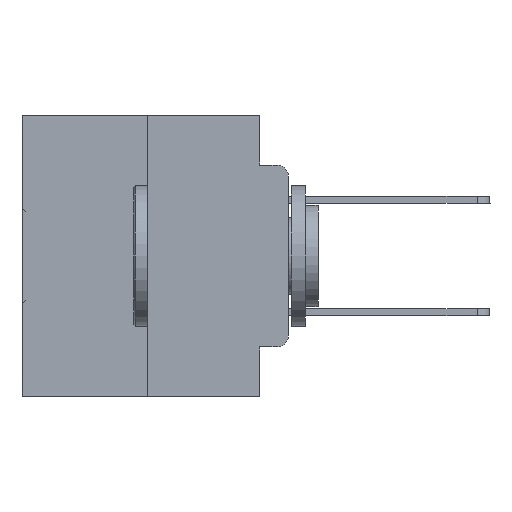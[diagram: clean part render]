
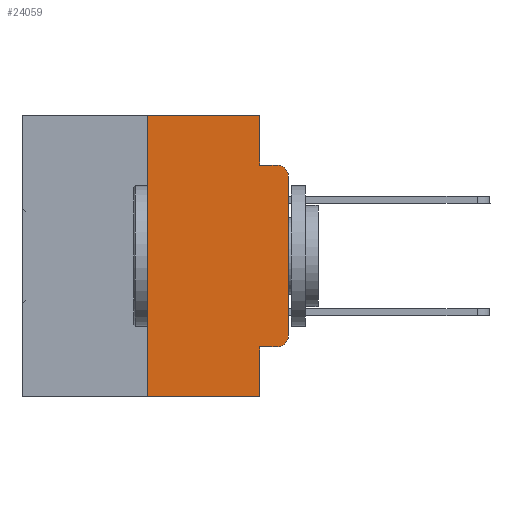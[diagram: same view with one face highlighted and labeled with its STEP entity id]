
A CAD part, left-side view. The second image highlights one B-rep face of the part: STEP entity #24059.
In plain terms, the highlighted planar face has unit normal (-1, 0, 0).
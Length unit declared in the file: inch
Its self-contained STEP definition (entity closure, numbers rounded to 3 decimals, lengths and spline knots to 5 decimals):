
#726 = EDGE_LOOP ( 'NONE', ( #24834, #34474, #28159, #8628, #19792, #15098, #16717, #9718, #22129, #34098 ) ) ;
#795 = EDGE_CURVE ( 'NONE', #1581, #10799, #4745, .T. ) ;
#1581 = VERTEX_POINT ( 'NONE', #32515 ) ;
#2024 = CARTESIAN_POINT ( 'NONE',  ( 0., 0.473, 0. ) ) ;
#2047 = DIRECTION ( 'NONE',  ( -1., 0., 0. ) ) ;
#2384 = DIRECTION ( 'NONE',  ( -1., 0., 0. ) ) ;
#2944 = DIRECTION ( 'NONE',  ( 0., -1., 0. ) ) ;
#4261 = EDGE_CURVE ( 'NONE', #22751, #6468, #29670, .T. ) ;
#4745 = LINE ( 'NONE', #30474, #30643 ) ;
#4764 = CARTESIAN_POINT ( 'NONE',  ( 0., 0.051, -0.4115 ) ) ;
#4934 = FACE_OUTER_BOUND ( 'NONE', #726, .T. ) ;
#5208 = CIRCLE ( 'NONE', #13096, 0.02 ) ;
#5862 = EDGE_CURVE ( 'NONE', #1581, #19185, #18358, .T. ) ;
#6235 = VERTEX_POINT ( 'NONE', #17191 ) ;
#6460 = CIRCLE ( 'NONE', #14103, 0.02 ) ;
#6468 = VERTEX_POINT ( 'NONE', #27040 ) ;
#6824 = EDGE_CURVE ( 'NONE', #12657, #6235, #22444, .T. ) ;
#8425 = LINE ( 'NONE', #23214, #25607 ) ;
#8628 = ORIENTED_EDGE ( 'NONE', *, *, #6824, .F. ) ;
#9556 = DIRECTION ( 'NONE',  ( 0., -1., 0. ) ) ;
#9718 = ORIENTED_EDGE ( 'NONE', *, *, #28615, .F. ) ;
#9934 = VECTOR ( 'NONE', #9556, 39.37008 ) ;
#10799 = VERTEX_POINT ( 'NONE', #25189 ) ;
#10883 = CARTESIAN_POINT ( 'NONE',  ( 0., 0.051, -0.5 ) ) ;
#11021 = CARTESIAN_POINT ( 'NONE',  ( 0., 0.473, -0.5 ) ) ;
#11937 = VECTOR ( 'NONE', #12017, 39.37008 ) ;
#12017 = DIRECTION ( 'NONE',  ( 0., 0., -1. ) ) ;
#12071 = DIRECTION ( 'NONE',  ( 0., -1., 0. ) ) ;
#12657 = VERTEX_POINT ( 'NONE', #19459 ) ;
#12986 = LINE ( 'NONE', #22172, #19304 ) ;
#13096 = AXIS2_PLACEMENT_3D ( 'NONE', #21367, #2384, #29260 ) ;
#14103 = AXIS2_PLACEMENT_3D ( 'NONE', #23578, #2047, #28794 ) ;
#14112 = VECTOR ( 'NONE', #2944, 39.37008 ) ;
#14984 = CARTESIAN_POINT ( 'NONE',  ( 0., 0., 0. ) ) ;
#15098 = ORIENTED_EDGE ( 'NONE', *, *, #795, .F. ) ;
#15386 = DIRECTION ( 'NONE',  ( 1., 0., 0. ) ) ;
#16717 = ORIENTED_EDGE ( 'NONE', *, *, #5862, .T. ) ;
#17191 = CARTESIAN_POINT ( 'NONE',  ( 0., 0.051, -0.0885 ) ) ;
#18059 = VECTOR ( 'NONE', #29953, 39.37008 ) ;
#18358 = LINE ( 'NONE', #11021, #14112 ) ;
#18362 = EDGE_CURVE ( 'NONE', #10799, #12657, #12986, .T. ) ;
#18928 = AXIS2_PLACEMENT_3D ( 'NONE', #2024, #15386, #28770 ) ;
#19160 = LINE ( 'NONE', #4764, #9934 ) ;
#19185 = VERTEX_POINT ( 'NONE', #10883 ) ;
#19304 = VECTOR ( 'NONE', #27497, 39.37008 ) ;
#19459 = CARTESIAN_POINT ( 'NONE',  ( 0., 0.051, 0. ) ) ;
#19756 = EDGE_CURVE ( 'NONE', #22406, #20924, #19160, .T. ) ;
#19792 = ORIENTED_EDGE ( 'NONE', *, *, #18362, .F. ) ;
#20627 = DIRECTION ( 'NONE',  ( 0., 0., 1. ) ) ;
#20632 = CARTESIAN_POINT ( 'NONE',  ( 0., 0., -0.3915 ) ) ;
#20924 = VERTEX_POINT ( 'NONE', #25853 ) ;
#21367 = CARTESIAN_POINT ( 'NONE',  ( 0., 0.02, -0.1085 ) ) ;
#21571 = CARTESIAN_POINT ( 'NONE',  ( 0., 0.051, -0.4115 ) ) ;
#22103 = EDGE_CURVE ( 'NONE', #6235, #28125, #8425, .T. ) ;
#22129 = ORIENTED_EDGE ( 'NONE', *, *, #19756, .T. ) ;
#22172 = CARTESIAN_POINT ( 'NONE',  ( 0., 0.473, 0. ) ) ;
#22406 = VERTEX_POINT ( 'NONE', #21571 ) ;
#22444 = LINE ( 'NONE', #25363, #11937 ) ;
#22751 = VERTEX_POINT ( 'NONE', #20632 ) ;
#23120 = CARTESIAN_POINT ( 'NONE',  ( 0., 0.02, -0.0885 ) ) ;
#23214 = CARTESIAN_POINT ( 'NONE',  ( 0., 0.051, -0.0885 ) ) ;
#23578 = CARTESIAN_POINT ( 'NONE',  ( 0., 0.02, -0.3915 ) ) ;
#23911 = LINE ( 'NONE', #27272, #18059 ) ;
#24059 = ADVANCED_FACE ( 'NONE', ( #4934 ), #33652, .F. ) ;
#24834 = ORIENTED_EDGE ( 'NONE', *, *, #4261, .T. ) ;
#25139 = DIRECTION ( 'NONE',  ( 0., 0., 1. ) ) ;
#25189 = CARTESIAN_POINT ( 'NONE',  ( 0., 0.25, 0. ) ) ;
#25363 = CARTESIAN_POINT ( 'NONE',  ( 0., 0.051, 0. ) ) ;
#25607 = VECTOR ( 'NONE', #12071, 39.37008 ) ;
#25853 = CARTESIAN_POINT ( 'NONE',  ( 0., 0.02, -0.4115 ) ) ;
#26089 = EDGE_CURVE ( 'NONE', #6468, #28125, #5208, .T. ) ;
#27040 = CARTESIAN_POINT ( 'NONE',  ( 0., 0., -0.1085 ) ) ;
#27272 = CARTESIAN_POINT ( 'NONE',  ( 0., 0.051, 0. ) ) ;
#27497 = DIRECTION ( 'NONE',  ( 0., -1., 0. ) ) ;
#28125 = VERTEX_POINT ( 'NONE', #23120 ) ;
#28159 = ORIENTED_EDGE ( 'NONE', *, *, #22103, .F. ) ;
#28615 = EDGE_CURVE ( 'NONE', #22406, #19185, #23911, .T. ) ;
#28770 = DIRECTION ( 'NONE',  ( 0., 0., -1. ) ) ;
#28794 = DIRECTION ( 'NONE',  ( 0., 0., -1. ) ) ;
#29260 = DIRECTION ( 'NONE',  ( 0., 0., -1. ) ) ;
#29670 = LINE ( 'NONE', #14984, #32568 ) ;
#29953 = DIRECTION ( 'NONE',  ( 0., 0., -1. ) ) ;
#30474 = CARTESIAN_POINT ( 'NONE',  ( 0., 0.25, 0. ) ) ;
#30643 = VECTOR ( 'NONE', #25139, 39.37008 ) ;
#32015 = EDGE_CURVE ( 'NONE', #20924, #22751, #6460, .T. ) ;
#32515 = CARTESIAN_POINT ( 'NONE',  ( 0., 0.25, -0.5 ) ) ;
#32568 = VECTOR ( 'NONE', #20627, 39.37008 ) ;
#33652 = PLANE ( 'NONE',  #18928 ) ;
#34098 = ORIENTED_EDGE ( 'NONE', *, *, #32015, .T. ) ;
#34474 = ORIENTED_EDGE ( 'NONE', *, *, #26089, .T. ) ;
